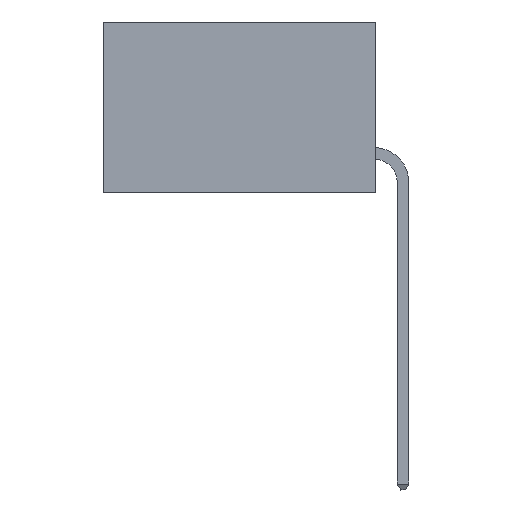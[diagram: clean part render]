
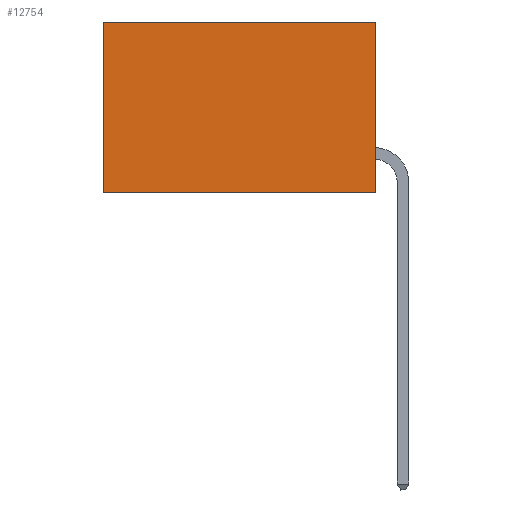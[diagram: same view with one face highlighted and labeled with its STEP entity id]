
A CAD part, left-side view. The second image highlights one B-rep face of the part: STEP entity #12754.
In plain terms, the highlighted planar face has unit normal (-1, 0, 0).
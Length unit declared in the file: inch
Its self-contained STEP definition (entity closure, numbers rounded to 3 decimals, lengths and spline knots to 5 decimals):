
#462 = CARTESIAN_POINT ( 'NONE',  ( 0.277, 0., -0.37 ) ) ;
#1616 = VECTOR ( 'NONE', #4523, 39.37008 ) ;
#1654 = EDGE_CURVE ( 'NONE', #1724, #6159, #7398, .T. ) ;
#1724 = VERTEX_POINT ( 'NONE', #13473 ) ;
#3415 = CARTESIAN_POINT ( 'NONE',  ( 0.277, 0., -0.37 ) ) ;
#3826 = DIRECTION ( 'NONE',  ( 0., 1., 0. ) ) ;
#3999 = CARTESIAN_POINT ( 'NONE',  ( 0.277, 0.59, -0.37 ) ) ;
#4326 = DIRECTION ( 'NONE',  ( 0., 0., -1. ) ) ;
#4336 = PLANE ( 'NONE',  #18517 ) ;
#4523 = DIRECTION ( 'NONE',  ( 0., 0., -1. ) ) ;
#4801 = ORIENTED_EDGE ( 'NONE', *, *, #17088, .F. ) ;
#4811 = CARTESIAN_POINT ( 'NONE',  ( 0.277, 0.59, -0.37 ) ) ;
#5020 = LINE ( 'NONE', #6262, #14556 ) ;
#6159 = VERTEX_POINT ( 'NONE', #6822 ) ;
#6262 = CARTESIAN_POINT ( 'NONE',  ( 0.277, 0., -0.37 ) ) ;
#6275 = DIRECTION ( 'NONE',  ( 1., 0., 0. ) ) ;
#6822 = CARTESIAN_POINT ( 'NONE',  ( 0.277, 0.59, 0. ) ) ;
#7373 = EDGE_CURVE ( 'NONE', #6159, #14969, #16806, .T. ) ;
#7398 = LINE ( 'NONE', #8009, #16830 ) ;
#8009 = CARTESIAN_POINT ( 'NONE',  ( 0.277, 0., 0. ) ) ;
#8078 = ORIENTED_EDGE ( 'NONE', *, *, #20177, .F. ) ;
#8145 = DIRECTION ( 'NONE',  ( 0., 1., 0. ) ) ;
#9408 = VECTOR ( 'NONE', #3826, 39.37008 ) ;
#11696 = ORIENTED_EDGE ( 'NONE', *, *, #1654, .T. ) ;
#12754 = ADVANCED_FACE ( 'NONE', ( #17380 ), #4336, .F. ) ;
#13346 = CARTESIAN_POINT ( 'NONE',  ( 0.277, 0., -0.37 ) ) ;
#13473 = CARTESIAN_POINT ( 'NONE',  ( 0.277, 0., 0. ) ) ;
#14446 = LINE ( 'NONE', #13346, #9408 ) ;
#14556 = VECTOR ( 'NONE', #4326, 39.37008 ) ;
#14811 = VERTEX_POINT ( 'NONE', #3415 ) ;
#14969 = VERTEX_POINT ( 'NONE', #3999 ) ;
#16806 = LINE ( 'NONE', #4811, #1616 ) ;
#16830 = VECTOR ( 'NONE', #8145, 39.37008 ) ;
#17088 = EDGE_CURVE ( 'NONE', #1724, #14811, #5020, .T. ) ;
#17380 = FACE_OUTER_BOUND ( 'NONE', #18538, .T. ) ;
#18517 = AXIS2_PLACEMENT_3D ( 'NONE', #462, #6275, #19445 ) ;
#18538 = EDGE_LOOP ( 'NONE', ( #22069, #8078, #4801, #11696 ) ) ;
#19445 = DIRECTION ( 'NONE',  ( 0., 0., -1. ) ) ;
#20177 = EDGE_CURVE ( 'NONE', #14811, #14969, #14446, .T. ) ;
#22069 = ORIENTED_EDGE ( 'NONE', *, *, #7373, .T. ) ;
